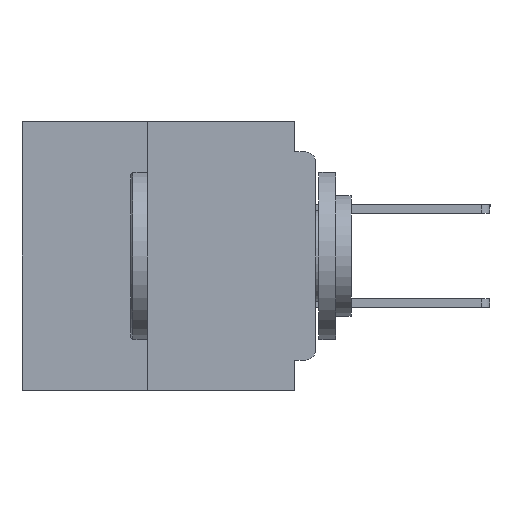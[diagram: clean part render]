
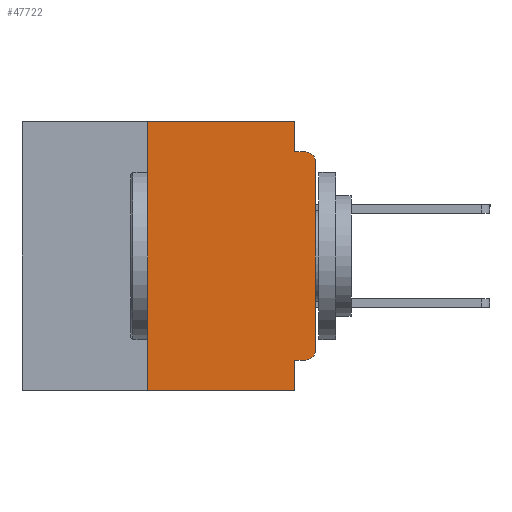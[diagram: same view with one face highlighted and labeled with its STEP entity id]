
A CAD part, left-side view. The second image highlights one B-rep face of the part: STEP entity #47722.
In plain terms, the highlighted planar face has unit normal (-1, 0, 0).
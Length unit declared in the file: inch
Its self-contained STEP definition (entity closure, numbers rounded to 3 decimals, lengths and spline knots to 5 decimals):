
#134 = VECTOR ( 'NONE', #50658, 39.37008 ) ;
#152 = VERTEX_POINT ( 'NONE', #40540 ) ;
#522 = EDGE_CURVE ( 'NONE', #44350, #42987, #58686, .T. ) ;
#1089 = CARTESIAN_POINT ( 'NONE',  ( 0., 0.25, 0. ) ) ;
#1549 = VERTEX_POINT ( 'NONE', #16843 ) ;
#3078 = VECTOR ( 'NONE', #34654, 39.37008 ) ;
#5446 = CARTESIAN_POINT ( 'NONE',  ( 0., 0.031, -0.355 ) ) ;
#7529 = ORIENTED_EDGE ( 'NONE', *, *, #33587, .F. ) ;
#9202 = VECTOR ( 'NONE', #51393, 39.37008 ) ;
#9927 = DIRECTION ( 'NONE',  ( -1., 0., 0. ) ) ;
#10748 = AXIS2_PLACEMENT_3D ( 'NONE', #27241, #59817, #31963 ) ;
#11397 = VERTEX_POINT ( 'NONE', #51632 ) ;
#12105 = EDGE_CURVE ( 'NONE', #31481, #152, #31287, .T. ) ;
#12155 = VECTOR ( 'NONE', #60252, 39.37008 ) ;
#12610 = CARTESIAN_POINT ( 'NONE',  ( 0., 0.031, -0.4 ) ) ;
#13305 = ORIENTED_EDGE ( 'NONE', *, *, #33681, .T. ) ;
#15119 = EDGE_CURVE ( 'NONE', #152, #1549, #37529, .T. ) ;
#16843 = CARTESIAN_POINT ( 'NONE',  ( 0., 0., -0.06 ) ) ;
#17811 = ORIENTED_EDGE ( 'NONE', *, *, #24770, .T. ) ;
#19878 = ORIENTED_EDGE ( 'NONE', *, *, #27283, .F. ) ;
#20216 = VERTEX_POINT ( 'NONE', #1089 ) ;
#20835 = VERTEX_POINT ( 'NONE', #48021 ) ;
#22370 = CARTESIAN_POINT ( 'NONE',  ( 0., 0., -0.355 ) ) ;
#23785 = EDGE_CURVE ( 'NONE', #28817, #11397, #37437, .T. ) ;
#24625 = LINE ( 'NONE', #50910, #60313 ) ;
#24770 = EDGE_CURVE ( 'NONE', #1549, #28191, #51898, .T. ) ;
#25470 = CARTESIAN_POINT ( 'NONE',  ( 0., 0.015, -0.06 ) ) ;
#26044 = LINE ( 'NONE', #41714, #12155 ) ;
#26398 = ORIENTED_EDGE ( 'NONE', *, *, #12105, .T. ) ;
#27241 = CARTESIAN_POINT ( 'NONE',  ( 0., 0.437, 0. ) ) ;
#27283 = EDGE_CURVE ( 'NONE', #20216, #28817, #46481, .T. ) ;
#28191 = VERTEX_POINT ( 'NONE', #54150 ) ;
#28817 = VERTEX_POINT ( 'NONE', #53344 ) ;
#29045 = VECTOR ( 'NONE', #40899, 39.37008 ) ;
#29521 = LINE ( 'NONE', #58049, #3078 ) ;
#30195 = DIRECTION ( 'NONE',  ( 0., 0., -1. ) ) ;
#31287 = CIRCLE ( 'NONE', #46699, 0.015 ) ;
#31481 = VERTEX_POINT ( 'NONE', #39318 ) ;
#31963 = DIRECTION ( 'NONE',  ( 0., 0., -1. ) ) ;
#32483 = CARTESIAN_POINT ( 'NONE',  ( 0., 0.437, 0. ) ) ;
#33587 = EDGE_CURVE ( 'NONE', #31481, #44350, #53759, .T. ) ;
#33681 = EDGE_CURVE ( 'NONE', #20835, #42987, #24625, .T. ) ;
#33689 = EDGE_CURVE ( 'NONE', #20835, #20216, #26044, .T. ) ;
#33751 = FACE_OUTER_BOUND ( 'NONE', #45431, .T. ) ;
#33934 = VECTOR ( 'NONE', #39851, 39.37008 ) ;
#34654 = DIRECTION ( 'NONE',  ( 0., -1., 0. ) ) ;
#37049 = CARTESIAN_POINT ( 'NONE',  ( 0., 0.031, -0.4 ) ) ;
#37437 = LINE ( 'NONE', #46198, #134 ) ;
#37529 = LINE ( 'NONE', #53761, #47008 ) ;
#37905 = CARTESIAN_POINT ( 'NONE',  ( 0., 0.015, -0.34 ) ) ;
#39318 = CARTESIAN_POINT ( 'NONE',  ( 0., 0.015, -0.355 ) ) ;
#39851 = DIRECTION ( 'NONE',  ( 0., 0., -1. ) ) ;
#40540 = CARTESIAN_POINT ( 'NONE',  ( 0., 0., -0.34 ) ) ;
#40899 = DIRECTION ( 'NONE',  ( 0., 1., 0. ) ) ;
#41506 = DIRECTION ( 'NONE',  ( 0., -1., 0. ) ) ;
#41714 = CARTESIAN_POINT ( 'NONE',  ( 0., 0.25, -0.4 ) ) ;
#42578 = DIRECTION ( 'NONE',  ( 0., 0., -1. ) ) ;
#42987 = VERTEX_POINT ( 'NONE', #37049 ) ;
#44350 = VERTEX_POINT ( 'NONE', #5446 ) ;
#44429 = ORIENTED_EDGE ( 'NONE', *, *, #15119, .T. ) ;
#45431 = EDGE_LOOP ( 'NONE', ( #44429, #17811, #52084, #53227, #19878, #58123, #13305, #51788, #7529, #26398 ) ) ;
#46198 = CARTESIAN_POINT ( 'NONE',  ( 0., 0.031, 0. ) ) ;
#46481 = LINE ( 'NONE', #32483, #9202 ) ;
#46699 = AXIS2_PLACEMENT_3D ( 'NONE', #37905, #9927, #42578 ) ;
#47008 = VECTOR ( 'NONE', #49080, 39.37008 ) ;
#47478 = AXIS2_PLACEMENT_3D ( 'NONE', #25470, #58053, #30195 ) ;
#47722 = ADVANCED_FACE ( 'NONE', ( #33751 ), #55151, .F. ) ;
#48021 = CARTESIAN_POINT ( 'NONE',  ( 0., 0.25, -0.4 ) ) ;
#49080 = DIRECTION ( 'NONE',  ( 0., 0., 1. ) ) ;
#50658 = DIRECTION ( 'NONE',  ( 0., 0., -1. ) ) ;
#50910 = CARTESIAN_POINT ( 'NONE',  ( 0., 0.437, -0.4 ) ) ;
#51393 = DIRECTION ( 'NONE',  ( 0., -1., 0. ) ) ;
#51632 = CARTESIAN_POINT ( 'NONE',  ( 0., 0.031, -0.045 ) ) ;
#51788 = ORIENTED_EDGE ( 'NONE', *, *, #522, .F. ) ;
#51898 = CIRCLE ( 'NONE', #47478, 0.015 ) ;
#52084 = ORIENTED_EDGE ( 'NONE', *, *, #58538, .F. ) ;
#53227 = ORIENTED_EDGE ( 'NONE', *, *, #23785, .F. ) ;
#53344 = CARTESIAN_POINT ( 'NONE',  ( 0., 0.031, 0. ) ) ;
#53759 = LINE ( 'NONE', #22370, #29045 ) ;
#53761 = CARTESIAN_POINT ( 'NONE',  ( 0., 0., 0. ) ) ;
#54150 = CARTESIAN_POINT ( 'NONE',  ( 0., 0.015, -0.045 ) ) ;
#55151 = PLANE ( 'NONE',  #10748 ) ;
#58049 = CARTESIAN_POINT ( 'NONE',  ( 0., 0., -0.045 ) ) ;
#58053 = DIRECTION ( 'NONE',  ( -1., 0., 0. ) ) ;
#58123 = ORIENTED_EDGE ( 'NONE', *, *, #33689, .F. ) ;
#58538 = EDGE_CURVE ( 'NONE', #11397, #28191, #29521, .T. ) ;
#58686 = LINE ( 'NONE', #12610, #33934 ) ;
#59817 = DIRECTION ( 'NONE',  ( 1., 0., 0. ) ) ;
#60252 = DIRECTION ( 'NONE',  ( 0., 0., 1. ) ) ;
#60313 = VECTOR ( 'NONE', #41506, 39.37008 ) ;
